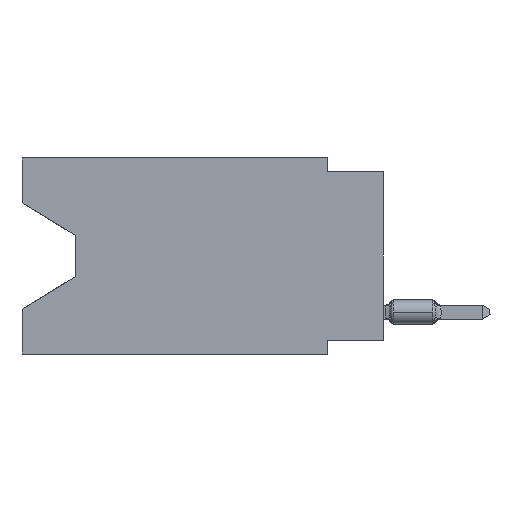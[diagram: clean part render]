
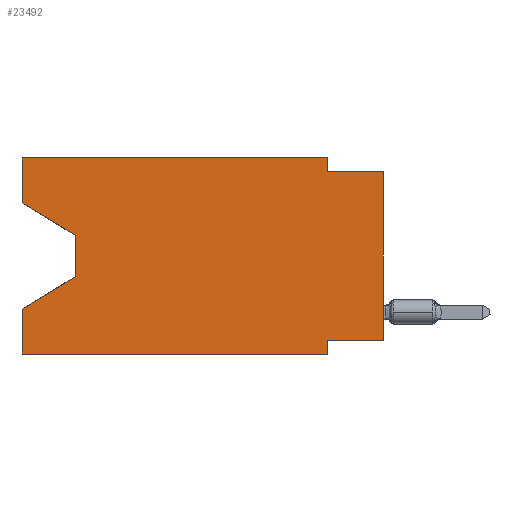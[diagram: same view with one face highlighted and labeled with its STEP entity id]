
A CAD part, left-side view. The second image highlights one B-rep face of the part: STEP entity #23492.
In plain terms, the highlighted planar face has unit normal (-1, 0, 0).
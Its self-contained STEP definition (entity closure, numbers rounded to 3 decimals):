
#1677 = ORIENTED_EDGE ( 'NONE', *, *, #47517, .T. ) ;
#1930 = DIRECTION ( 'NONE',  ( 0., 0., -1. ) ) ;
#3000 = CARTESIAN_POINT ( 'NONE',  ( 0., 13.97, -3.505 ) ) ;
#3228 = EDGE_CURVE ( 'NONE', #34355, #18461, #10208, .T. ) ;
#3727 = LINE ( 'NONE', #40762, #29760 ) ;
#4629 = DIRECTION ( 'NONE',  ( 0., -1., 0. ) ) ;
#4883 = CARTESIAN_POINT ( 'NONE',  ( 0., 2.54, -8.89 ) ) ;
#5337 = LINE ( 'NONE', #12857, #9200 ) ;
#6051 = DIRECTION ( 'NONE',  ( 0., 0., 1. ) ) ;
#7081 = VERTEX_POINT ( 'NONE', #11723 ) ;
#7147 = CARTESIAN_POINT ( 'NONE',  ( 0., 16.383, -2.038 ) ) ;
#8372 = VECTOR ( 'NONE', #37753, 1000. ) ;
#9200 = VECTOR ( 'NONE', #1930, 1000. ) ;
#9492 = EDGE_CURVE ( 'NONE', #45995, #12780, #16866, .T. ) ;
#9689 = EDGE_CURVE ( 'NONE', #10321, #28654, #25619, .T. ) ;
#10208 = LINE ( 'NONE', #21406, #8372 ) ;
#10321 = VERTEX_POINT ( 'NONE', #38676 ) ;
#10969 = CARTESIAN_POINT ( 'NONE',  ( 0., 13.97, -3.505 ) ) ;
#11723 = CARTESIAN_POINT ( 'NONE',  ( 0., 2.54, -0.635 ) ) ;
#11975 = CARTESIAN_POINT ( 'NONE',  ( 0., 2.54, -8.255 ) ) ;
#12006 = ORIENTED_EDGE ( 'NONE', *, *, #44504, .F. ) ;
#12780 = VERTEX_POINT ( 'NONE', #36884 ) ;
#12857 = CARTESIAN_POINT ( 'NONE',  ( 0., 2.54, 0. ) ) ;
#14017 = VERTEX_POINT ( 'NONE', #10969 ) ;
#14182 = DIRECTION ( 'NONE',  ( 0., 0., -1. ) ) ;
#14233 = DIRECTION ( 'NONE',  ( 0., -0.855, -0.519 ) ) ;
#14658 = FACE_OUTER_BOUND ( 'NONE', #22255, .T. ) ;
#14914 = VECTOR ( 'NONE', #24190, 1000. ) ;
#15540 = VECTOR ( 'NONE', #4629, 1000. ) ;
#16326 = VECTOR ( 'NONE', #37061, 1000. ) ;
#16866 = LINE ( 'NONE', #20534, #14914 ) ;
#16933 = CARTESIAN_POINT ( 'NONE',  ( 0., 16.383, -2.038 ) ) ;
#17414 = LINE ( 'NONE', #33012, #18927 ) ;
#17826 = CARTESIAN_POINT ( 'NONE',  ( 0., 16.383, 0. ) ) ;
#18461 = VERTEX_POINT ( 'NONE', #4883 ) ;
#18927 = VECTOR ( 'NONE', #28161, 1000. ) ;
#19211 = VECTOR ( 'NONE', #14233, 1000. ) ;
#19277 = CARTESIAN_POINT ( 'NONE',  ( 0., 16.383, -6.852 ) ) ;
#20270 = ORIENTED_EDGE ( 'NONE', *, *, #3228, .F. ) ;
#20534 = CARTESIAN_POINT ( 'NONE',  ( 0., 0., 0. ) ) ;
#21406 = CARTESIAN_POINT ( 'NONE',  ( 0., 2.54, -8.89 ) ) ;
#21967 = CARTESIAN_POINT ( 'NONE',  ( 0., 13.97, -5.385 ) ) ;
#22255 = EDGE_LOOP ( 'NONE', ( #1677, #39353, #37046, #45692, #35137, #20270, #12006, #47874, #43592, #42290, #27412, #29146 ) ) ;
#22690 = VERTEX_POINT ( 'NONE', #7147 ) ;
#23492 = ADVANCED_FACE ( 'NONE', ( #14658 ), #36373, .F. ) ;
#23967 = EDGE_CURVE ( 'NONE', #45866, #18461, #42144, .T. ) ;
#24086 = LINE ( 'NONE', #35088, #29621 ) ;
#24190 = DIRECTION ( 'NONE',  ( 0., 0., 1. ) ) ;
#24912 = DIRECTION ( 'NONE',  ( 0., 0., -1. ) ) ;
#25619 = LINE ( 'NONE', #21967, #33645 ) ;
#26092 = CARTESIAN_POINT ( 'NONE',  ( 0., 0., -8.255 ) ) ;
#26694 = DIRECTION ( 'NONE',  ( 0., -1., 0. ) ) ;
#26986 = CARTESIAN_POINT ( 'NONE',  ( 0., 2.54, 0. ) ) ;
#27412 = ORIENTED_EDGE ( 'NONE', *, *, #42583, .F. ) ;
#28161 = DIRECTION ( 'NONE',  ( 0., 0., 1. ) ) ;
#28654 = VERTEX_POINT ( 'NONE', #19277 ) ;
#29146 = ORIENTED_EDGE ( 'NONE', *, *, #38565, .F. ) ;
#29294 = DIRECTION ( 'NONE',  ( 0., -1., 0. ) ) ;
#29621 = VECTOR ( 'NONE', #6051, 1000. ) ;
#29760 = VECTOR ( 'NONE', #29294, 1000. ) ;
#30305 = AXIS2_PLACEMENT_3D ( 'NONE', #17826, #32709, #14182 ) ;
#30604 = EDGE_CURVE ( 'NONE', #7081, #12780, #3727, .T. ) ;
#31896 = EDGE_CURVE ( 'NONE', #45866, #28654, #17414, .T. ) ;
#32709 = DIRECTION ( 'NONE',  ( 1., 0., 0. ) ) ;
#33012 = CARTESIAN_POINT ( 'NONE',  ( 0., 16.383, 0. ) ) ;
#33645 = VECTOR ( 'NONE', #47568, 1000. ) ;
#34254 = LINE ( 'NONE', #34500, #38460 ) ;
#34355 = VERTEX_POINT ( 'NONE', #11975 ) ;
#34500 = CARTESIAN_POINT ( 'NONE',  ( 0., 16.383, 0. ) ) ;
#35088 = CARTESIAN_POINT ( 'NONE',  ( 0., 16.383, 0. ) ) ;
#35137 = ORIENTED_EDGE ( 'NONE', *, *, #23967, .T. ) ;
#35764 = CARTESIAN_POINT ( 'NONE',  ( 0., 16.383, -8.89 ) ) ;
#36373 = PLANE ( 'NONE',  #30305 ) ;
#36869 = LINE ( 'NONE', #3000, #46154 ) ;
#36884 = CARTESIAN_POINT ( 'NONE',  ( 0., 0., -0.635 ) ) ;
#37046 = ORIENTED_EDGE ( 'NONE', *, *, #9689, .T. ) ;
#37061 = DIRECTION ( 'NONE',  ( 0., 1., 0. ) ) ;
#37753 = DIRECTION ( 'NONE',  ( 0., 0., -1. ) ) ;
#38460 = VECTOR ( 'NONE', #26694, 1000. ) ;
#38565 = EDGE_CURVE ( 'NONE', #22690, #43207, #24086, .T. ) ;
#38676 = CARTESIAN_POINT ( 'NONE',  ( 0., 13.97, -5.385 ) ) ;
#39353 = ORIENTED_EDGE ( 'NONE', *, *, #41073, .T. ) ;
#40079 = LINE ( 'NONE', #16933, #19211 ) ;
#40762 = CARTESIAN_POINT ( 'NONE',  ( 0., 0., -0.635 ) ) ;
#41073 = EDGE_CURVE ( 'NONE', #14017, #10321, #36869, .T. ) ;
#42144 = LINE ( 'NONE', #46514, #15540 ) ;
#42290 = ORIENTED_EDGE ( 'NONE', *, *, #48192, .F. ) ;
#42583 = EDGE_CURVE ( 'NONE', #43207, #43444, #34254, .T. ) ;
#43207 = VERTEX_POINT ( 'NONE', #45286 ) ;
#43444 = VERTEX_POINT ( 'NONE', #26986 ) ;
#43592 = ORIENTED_EDGE ( 'NONE', *, *, #30604, .F. ) ;
#44030 = CARTESIAN_POINT ( 'NONE',  ( 0., 0., -8.255 ) ) ;
#44504 = EDGE_CURVE ( 'NONE', #45995, #34355, #44631, .T. ) ;
#44631 = LINE ( 'NONE', #26092, #16326 ) ;
#45286 = CARTESIAN_POINT ( 'NONE',  ( 0., 16.383, 0. ) ) ;
#45692 = ORIENTED_EDGE ( 'NONE', *, *, #31896, .F. ) ;
#45866 = VERTEX_POINT ( 'NONE', #35764 ) ;
#45995 = VERTEX_POINT ( 'NONE', #44030 ) ;
#46154 = VECTOR ( 'NONE', #24912, 1000. ) ;
#46514 = CARTESIAN_POINT ( 'NONE',  ( 0., 16.383, -8.89 ) ) ;
#47517 = EDGE_CURVE ( 'NONE', #22690, #14017, #40079, .T. ) ;
#47568 = DIRECTION ( 'NONE',  ( 0., 0.855, -0.519 ) ) ;
#47874 = ORIENTED_EDGE ( 'NONE', *, *, #9492, .T. ) ;
#48192 = EDGE_CURVE ( 'NONE', #43444, #7081, #5337, .T. ) ;
